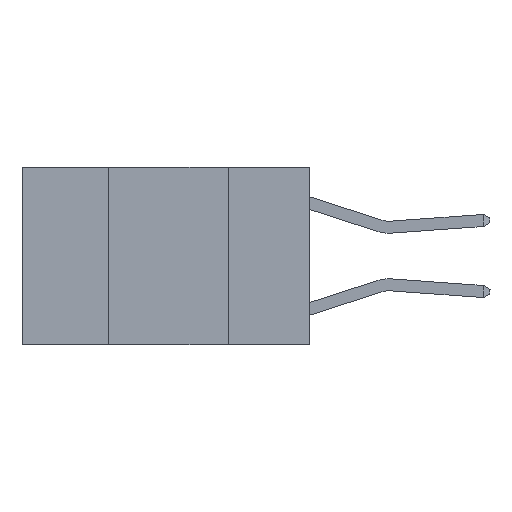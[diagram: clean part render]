
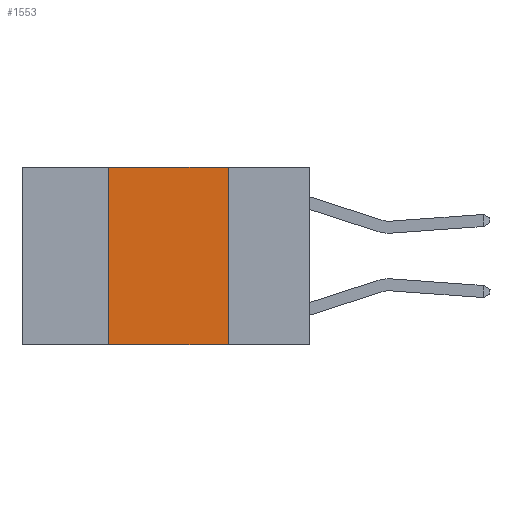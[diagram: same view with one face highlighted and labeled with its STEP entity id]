
A CAD part, left-side view. The second image highlights one B-rep face of the part: STEP entity #1553.
In plain terms, the highlighted planar face has unit normal (-1, 0, 0).
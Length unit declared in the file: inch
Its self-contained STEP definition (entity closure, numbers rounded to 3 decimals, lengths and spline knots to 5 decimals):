
#192 = PLANE ( 'NONE',  #7074 ) ;
#879 = DIRECTION ( 'NONE',  ( 0., 0., 1. ) ) ;
#1130 = EDGE_LOOP ( 'NONE', ( #3195, #1384, #3437, #5547 ) ) ;
#1156 = EDGE_CURVE ( 'NONE', #3558, #2092, #9387, .T. ) ;
#1254 = VECTOR ( 'NONE', #7504, 39.37008 ) ;
#1384 = ORIENTED_EDGE ( 'NONE', *, *, #9330, .F. ) ;
#1553 = ADVANCED_FACE ( 'NONE', ( #2113 ), #192, .F. ) ;
#1644 = EDGE_CURVE ( 'NONE', #7217, #8334, #3198, .T. ) ;
#1777 = DIRECTION ( 'NONE',  ( 1., 0., 0. ) ) ;
#2092 = VERTEX_POINT ( 'NONE', #8080 ) ;
#2113 = FACE_OUTER_BOUND ( 'NONE', #1130, .T. ) ;
#2300 = EDGE_CURVE ( 'NONE', #3558, #8334, #7445, .T. ) ;
#3195 = ORIENTED_EDGE ( 'NONE', *, *, #1644, .F. ) ;
#3198 = LINE ( 'NONE', #8943, #7341 ) ;
#3437 = ORIENTED_EDGE ( 'NONE', *, *, #1156, .F. ) ;
#3453 = VECTOR ( 'NONE', #879, 39.37008 ) ;
#3558 = VERTEX_POINT ( 'NONE', #9443 ) ;
#3942 = CARTESIAN_POINT ( 'NONE',  ( 0., 0.17, -0.37 ) ) ;
#4694 = LINE ( 'NONE', #9873, #4956 ) ;
#4956 = VECTOR ( 'NONE', #7560, 39.37008 ) ;
#5251 = CARTESIAN_POINT ( 'NONE',  ( 0., 0.6, 0. ) ) ;
#5477 = DIRECTION ( 'NONE',  ( 0., 0., -1. ) ) ;
#5547 = ORIENTED_EDGE ( 'NONE', *, *, #2300, .T. ) ;
#7074 = AXIS2_PLACEMENT_3D ( 'NONE', #5251, #1777, #8527 ) ;
#7217 = VERTEX_POINT ( 'NONE', #8938 ) ;
#7341 = VECTOR ( 'NONE', #5477, 39.37008 ) ;
#7445 = LINE ( 'NONE', #8892, #1254 ) ;
#7504 = DIRECTION ( 'NONE',  ( 0., -1., 0. ) ) ;
#7560 = DIRECTION ( 'NONE',  ( 0., -1., 0. ) ) ;
#8080 = CARTESIAN_POINT ( 'NONE',  ( 0., 0.42, 0. ) ) ;
#8334 = VERTEX_POINT ( 'NONE', #3942 ) ;
#8527 = DIRECTION ( 'NONE',  ( 0., 0., -1. ) ) ;
#8892 = CARTESIAN_POINT ( 'NONE',  ( 0., 0.6, -0.37 ) ) ;
#8938 = CARTESIAN_POINT ( 'NONE',  ( 0., 0.17, 0. ) ) ;
#8943 = CARTESIAN_POINT ( 'NONE',  ( 0., 0.17, 0. ) ) ;
#9330 = EDGE_CURVE ( 'NONE', #2092, #7217, #4694, .T. ) ;
#9387 = LINE ( 'NONE', #9439, #3453 ) ;
#9439 = CARTESIAN_POINT ( 'NONE',  ( 0., 0.42, 0. ) ) ;
#9443 = CARTESIAN_POINT ( 'NONE',  ( 0., 0.42, -0.37 ) ) ;
#9873 = CARTESIAN_POINT ( 'NONE',  ( 0., 0.6, 0. ) ) ;
